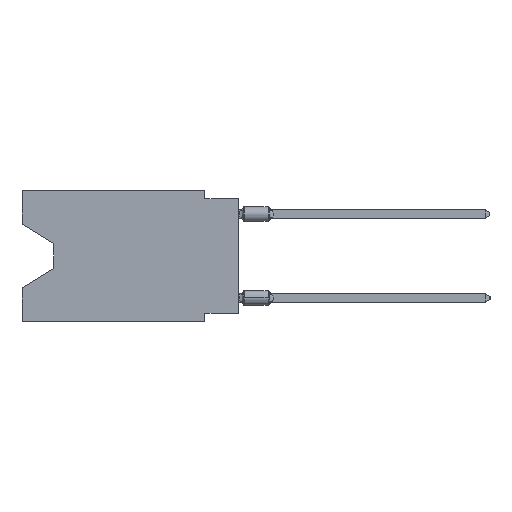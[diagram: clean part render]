
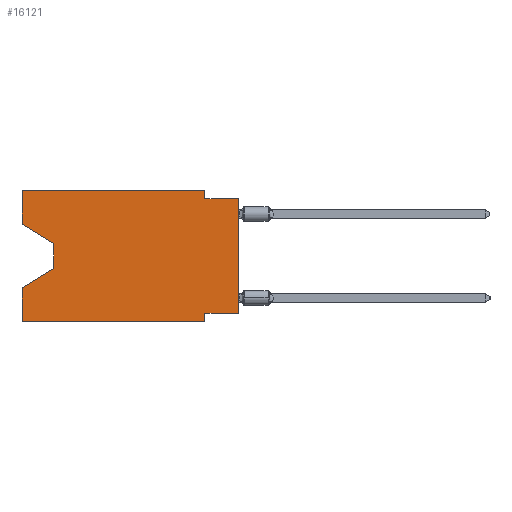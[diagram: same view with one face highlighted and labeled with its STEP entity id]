
A CAD part, left-side view. The second image highlights one B-rep face of the part: STEP entity #16121.
In plain terms, the highlighted planar face has unit normal (-1, 0, 0).
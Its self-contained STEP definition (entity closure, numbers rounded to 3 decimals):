
#214 = CARTESIAN_POINT ( 'NONE',  ( 0., 16.383, -2.546 ) ) ;
#374 = CARTESIAN_POINT ( 'NONE',  ( 0., 13.97, -5.893 ) ) ;
#572 = CARTESIAN_POINT ( 'NONE',  ( 0., 2.54, -9.271 ) ) ;
#847 = VECTOR ( 'NONE', #5734, 1000. ) ;
#1325 = EDGE_CURVE ( 'NONE', #30901, #13543, #8042, .T. ) ;
#1522 = ORIENTED_EDGE ( 'NONE', *, *, #12759, .F. ) ;
#1546 = CARTESIAN_POINT ( 'NONE',  ( 0., 16.383, -2.546 ) ) ;
#2155 = LINE ( 'NONE', #24888, #35441 ) ;
#2536 = DIRECTION ( 'NONE',  ( 0., -1., 0. ) ) ;
#2612 = CARTESIAN_POINT ( 'NONE',  ( 0., 16.383, -9.906 ) ) ;
#3603 = CARTESIAN_POINT ( 'NONE',  ( 0., 2.54, -9.906 ) ) ;
#3780 = VERTEX_POINT ( 'NONE', #25925 ) ;
#3869 = ORIENTED_EDGE ( 'NONE', *, *, #14568, .T. ) ;
#4180 = ORIENTED_EDGE ( 'NONE', *, *, #21037, .F. ) ;
#5039 = CARTESIAN_POINT ( 'NONE',  ( 0., 16.383, -9.906 ) ) ;
#5061 = CARTESIAN_POINT ( 'NONE',  ( 0., 0., -9.271 ) ) ;
#5346 = LINE ( 'NONE', #25467, #20411 ) ;
#5519 = DIRECTION ( 'NONE',  ( 0., 0., 1. ) ) ;
#5734 = DIRECTION ( 'NONE',  ( 0., 0., -1. ) ) ;
#6025 = CARTESIAN_POINT ( 'NONE',  ( 0., 2.54, 0. ) ) ;
#6087 = CARTESIAN_POINT ( 'NONE',  ( 0., 16.383, -7.36 ) ) ;
#6818 = LINE ( 'NONE', #15389, #21820 ) ;
#6885 = VECTOR ( 'NONE', #34695, 1000. ) ;
#7482 = EDGE_CURVE ( 'NONE', #13165, #28500, #17465, .T. ) ;
#8002 = ORIENTED_EDGE ( 'NONE', *, *, #7482, .F. ) ;
#8042 = LINE ( 'NONE', #5061, #9961 ) ;
#9433 = LINE ( 'NONE', #34383, #14550 ) ;
#9762 = DIRECTION ( 'NONE',  ( 0., -0.855, -0.519 ) ) ;
#9961 = VECTOR ( 'NONE', #36161, 1000. ) ;
#11422 = VERTEX_POINT ( 'NONE', #27105 ) ;
#12668 = ORIENTED_EDGE ( 'NONE', *, *, #20372, .F. ) ;
#12693 = AXIS2_PLACEMENT_3D ( 'NONE', #25551, #17735, #31871 ) ;
#12759 = EDGE_CURVE ( 'NONE', #31898, #13165, #9433, .T. ) ;
#13165 = VERTEX_POINT ( 'NONE', #6025 ) ;
#13178 = VERTEX_POINT ( 'NONE', #3603 ) ;
#13543 = VERTEX_POINT ( 'NONE', #572 ) ;
#14019 = PLANE ( 'NONE',  #12693 ) ;
#14550 = VECTOR ( 'NONE', #25816, 1000. ) ;
#14568 = EDGE_CURVE ( 'NONE', #3780, #11422, #32403, .T. ) ;
#15274 = VECTOR ( 'NONE', #5519, 1000. ) ;
#15389 = CARTESIAN_POINT ( 'NONE',  ( 0., 0., 0. ) ) ;
#15785 = ORIENTED_EDGE ( 'NONE', *, *, #25719, .T. ) ;
#16014 = CARTESIAN_POINT ( 'NONE',  ( 0., 2.54, -9.906 ) ) ;
#16121 = ADVANCED_FACE ( 'NONE', ( #31498 ), #14019, .F. ) ;
#16284 = VECTOR ( 'NONE', #27718, 1000. ) ;
#16831 = EDGE_CURVE ( 'NONE', #13543, #13178, #18990, .T. ) ;
#17465 = LINE ( 'NONE', #31233, #847 ) ;
#17735 = DIRECTION ( 'NONE',  ( 1., 0., 0. ) ) ;
#18075 = CARTESIAN_POINT ( 'NONE',  ( 0., 2.54, -0.635 ) ) ;
#18520 = VERTEX_POINT ( 'NONE', #23197 ) ;
#18763 = ORIENTED_EDGE ( 'NONE', *, *, #16831, .F. ) ;
#18990 = LINE ( 'NONE', #16014, #16284 ) ;
#19810 = CARTESIAN_POINT ( 'NONE',  ( 0., 13.97, -4.013 ) ) ;
#20271 = ORIENTED_EDGE ( 'NONE', *, *, #22227, .F. ) ;
#20372 = EDGE_CURVE ( 'NONE', #31359, #31898, #2155, .T. ) ;
#20411 = VECTOR ( 'NONE', #2536, 1000. ) ;
#21037 = EDGE_CURVE ( 'NONE', #33649, #27084, #22106, .T. ) ;
#21356 = DIRECTION ( 'NONE',  ( 0., 0., 1. ) ) ;
#21820 = VECTOR ( 'NONE', #21356, 1000. ) ;
#22106 = LINE ( 'NONE', #27497, #15274 ) ;
#22227 = EDGE_CURVE ( 'NONE', #28500, #18520, #5346, .T. ) ;
#22426 = VECTOR ( 'NONE', #9762, 1000. ) ;
#22934 = ORIENTED_EDGE ( 'NONE', *, *, #35004, .T. ) ;
#23197 = CARTESIAN_POINT ( 'NONE',  ( 0., 0., -0.635 ) ) ;
#24489 = VECTOR ( 'NONE', #28666, 1000. ) ;
#24569 = VECTOR ( 'NONE', #26073, 1000. ) ;
#24888 = CARTESIAN_POINT ( 'NONE',  ( 0., 16.383, 0. ) ) ;
#25265 = CARTESIAN_POINT ( 'NONE',  ( 0., 16.383, 0. ) ) ;
#25467 = CARTESIAN_POINT ( 'NONE',  ( 0., 0., -0.635 ) ) ;
#25551 = CARTESIAN_POINT ( 'NONE',  ( 0., 16.383, 0. ) ) ;
#25719 = EDGE_CURVE ( 'NONE', #30901, #18520, #6818, .T. ) ;
#25816 = DIRECTION ( 'NONE',  ( 0., -1., 0. ) ) ;
#25925 = CARTESIAN_POINT ( 'NONE',  ( 0., 13.97, -4.013 ) ) ;
#26073 = DIRECTION ( 'NONE',  ( 0., -1., 0. ) ) ;
#27084 = VERTEX_POINT ( 'NONE', #6087 ) ;
#27105 = CARTESIAN_POINT ( 'NONE',  ( 0., 13.97, -5.893 ) ) ;
#27366 = ORIENTED_EDGE ( 'NONE', *, *, #36325, .T. ) ;
#27457 = CARTESIAN_POINT ( 'NONE',  ( 0., 0., -9.271 ) ) ;
#27497 = CARTESIAN_POINT ( 'NONE',  ( 0., 16.383, 0. ) ) ;
#27646 = EDGE_CURVE ( 'NONE', #31359, #3780, #33023, .T. ) ;
#27718 = DIRECTION ( 'NONE',  ( 0., 0., -1. ) ) ;
#28500 = VERTEX_POINT ( 'NONE', #18075 ) ;
#28666 = DIRECTION ( 'NONE',  ( 0., 0.855, -0.519 ) ) ;
#30901 = VERTEX_POINT ( 'NONE', #27457 ) ;
#31233 = CARTESIAN_POINT ( 'NONE',  ( 0., 2.54, 0. ) ) ;
#31359 = VERTEX_POINT ( 'NONE', #214 ) ;
#31498 = FACE_OUTER_BOUND ( 'NONE', #33511, .T. ) ;
#31841 = LINE ( 'NONE', #374, #24489 ) ;
#31871 = DIRECTION ( 'NONE',  ( 0., 0., -1. ) ) ;
#31898 = VERTEX_POINT ( 'NONE', #25265 ) ;
#32197 = ORIENTED_EDGE ( 'NONE', *, *, #27646, .T. ) ;
#32403 = LINE ( 'NONE', #19810, #6885 ) ;
#33023 = LINE ( 'NONE', #1546, #22426 ) ;
#33511 = EDGE_LOOP ( 'NONE', ( #32197, #3869, #22934, #4180, #27366, #18763, #36428, #15785, #20271, #8002, #1522, #12668 ) ) ;
#33649 = VERTEX_POINT ( 'NONE', #5039 ) ;
#34383 = CARTESIAN_POINT ( 'NONE',  ( 0., 16.383, 0. ) ) ;
#34695 = DIRECTION ( 'NONE',  ( 0., 0., -1. ) ) ;
#35004 = EDGE_CURVE ( 'NONE', #11422, #27084, #31841, .T. ) ;
#35441 = VECTOR ( 'NONE', #36236, 1000. ) ;
#36161 = DIRECTION ( 'NONE',  ( 0., 1., 0. ) ) ;
#36236 = DIRECTION ( 'NONE',  ( 0., 0., 1. ) ) ;
#36325 = EDGE_CURVE ( 'NONE', #33649, #13178, #36692, .T. ) ;
#36428 = ORIENTED_EDGE ( 'NONE', *, *, #1325, .F. ) ;
#36692 = LINE ( 'NONE', #2612, #24569 ) ;
